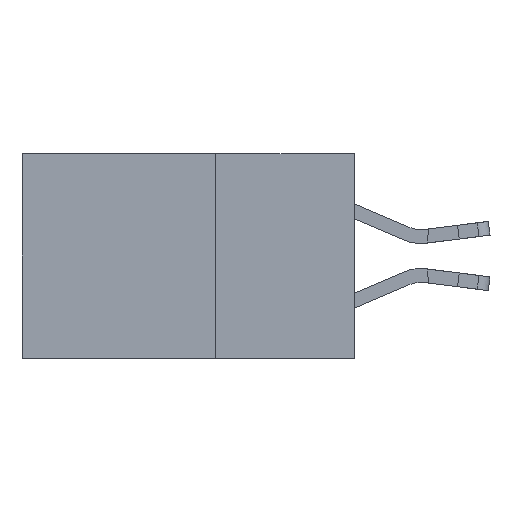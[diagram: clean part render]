
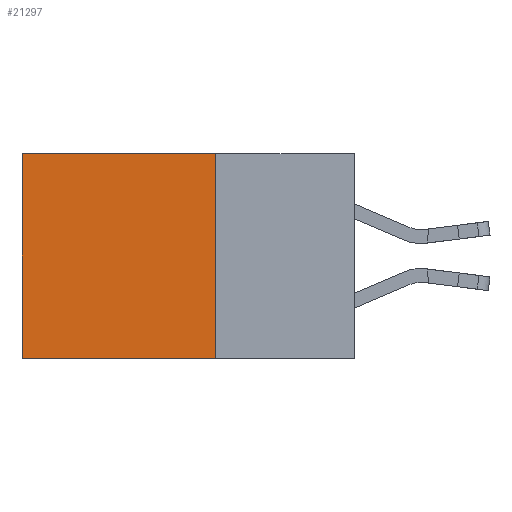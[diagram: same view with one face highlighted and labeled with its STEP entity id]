
A CAD part, left-side view. The second image highlights one B-rep face of the part: STEP entity #21297.
In plain terms, the highlighted planar face has unit normal (-1, 0, 0).
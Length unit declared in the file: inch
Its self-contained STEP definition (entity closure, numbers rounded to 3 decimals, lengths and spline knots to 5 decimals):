
#186 = LINE ( 'NONE', #19358, #22272 ) ;
#1500 = VECTOR ( 'NONE', #19313, 39.37008 ) ;
#2816 = VECTOR ( 'NONE', #20111, 39.37008 ) ;
#3080 = CARTESIAN_POINT ( 'NONE',  ( 0.298, 0.25, -0.37 ) ) ;
#3305 = AXIS2_PLACEMENT_3D ( 'NONE', #4005, #18914, #6186 ) ;
#4005 = CARTESIAN_POINT ( 'NONE',  ( 0.298, 0.25, 0. ) ) ;
#4431 = CARTESIAN_POINT ( 'NONE',  ( 0.298, 0.6, 0. ) ) ;
#4489 = DIRECTION ( 'NONE',  ( 0., 0., -1. ) ) ;
#4826 = CARTESIAN_POINT ( 'NONE',  ( 0.298, 0.6, -0.37 ) ) ;
#5001 = EDGE_CURVE ( 'NONE', #11783, #25232, #17359, .T. ) ;
#5190 = DIRECTION ( 'NONE',  ( 0., 1., 0. ) ) ;
#5358 = VECTOR ( 'NONE', #5190, 39.37008 ) ;
#5980 = CARTESIAN_POINT ( 'NONE',  ( 0.298, 0.25, 0. ) ) ;
#6186 = DIRECTION ( 'NONE',  ( 0., 0., -1. ) ) ;
#6626 = LINE ( 'NONE', #4431, #1500 ) ;
#7477 = VERTEX_POINT ( 'NONE', #12999 ) ;
#8288 = FACE_OUTER_BOUND ( 'NONE', #24424, .T. ) ;
#8771 = EDGE_CURVE ( 'NONE', #11783, #7477, #186, .T. ) ;
#11783 = VERTEX_POINT ( 'NONE', #5980 ) ;
#12546 = PLANE ( 'NONE',  #3305 ) ;
#12999 = CARTESIAN_POINT ( 'NONE',  ( 0.298, 0.25, -0.37 ) ) ;
#17359 = LINE ( 'NONE', #27232, #5358 ) ;
#17530 = CARTESIAN_POINT ( 'NONE',  ( 0.298, 0.6, 0. ) ) ;
#17624 = ORIENTED_EDGE ( 'NONE', *, *, #20707, .T. ) ;
#18627 = ORIENTED_EDGE ( 'NONE', *, *, #22585, .F. ) ;
#18914 = DIRECTION ( 'NONE',  ( 1., 0., 0. ) ) ;
#19313 = DIRECTION ( 'NONE',  ( 0., 0., -1. ) ) ;
#19358 = CARTESIAN_POINT ( 'NONE',  ( 0.298, 0.25, 0. ) ) ;
#20111 = DIRECTION ( 'NONE',  ( 0., 1., 0. ) ) ;
#20707 = EDGE_CURVE ( 'NONE', #25232, #26884, #6626, .T. ) ;
#21039 = ORIENTED_EDGE ( 'NONE', *, *, #5001, .T. ) ;
#21297 = ADVANCED_FACE ( 'NONE', ( #8288 ), #12546, .F. ) ;
#22272 = VECTOR ( 'NONE', #4489, 39.37008 ) ;
#22585 = EDGE_CURVE ( 'NONE', #7477, #26884, #26165, .T. ) ;
#24424 = EDGE_LOOP ( 'NONE', ( #17624, #18627, #26746, #21039 ) ) ;
#25232 = VERTEX_POINT ( 'NONE', #17530 ) ;
#26165 = LINE ( 'NONE', #3080, #2816 ) ;
#26746 = ORIENTED_EDGE ( 'NONE', *, *, #8771, .F. ) ;
#26884 = VERTEX_POINT ( 'NONE', #4826 ) ;
#27232 = CARTESIAN_POINT ( 'NONE',  ( 0.298, 0.25, 0. ) ) ;
